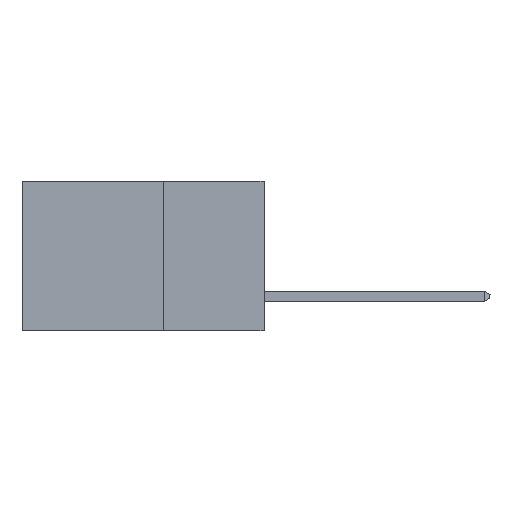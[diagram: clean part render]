
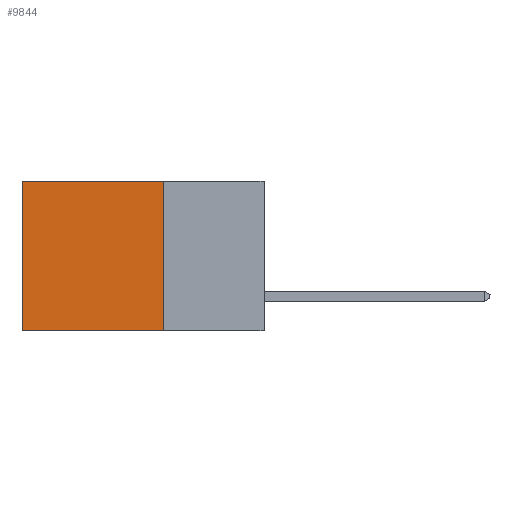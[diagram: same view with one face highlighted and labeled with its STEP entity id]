
A CAD part, left-side view. The second image highlights one B-rep face of the part: STEP entity #9844.
In plain terms, the highlighted planar face has unit normal (-1, 0, 0).
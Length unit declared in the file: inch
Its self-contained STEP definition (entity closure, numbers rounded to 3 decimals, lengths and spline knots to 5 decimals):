
#89 = ORIENTED_EDGE ( 'NONE', *, *, #6728, .F. ) ;
#309 = VERTEX_POINT ( 'NONE', #2510 ) ;
#455 = DIRECTION ( 'NONE',  ( 0., 0., -1. ) ) ;
#757 = DIRECTION ( 'NONE',  ( 0., 0., -1. ) ) ;
#859 = ORIENTED_EDGE ( 'NONE', *, *, #11018, .T. ) ;
#1404 = ORIENTED_EDGE ( 'NONE', *, *, #5015, .F. ) ;
#1527 = LINE ( 'NONE', #5231, #3447 ) ;
#2150 = CARTESIAN_POINT ( 'NONE',  ( 0.2615, 0.6, -0.37 ) ) ;
#2510 = CARTESIAN_POINT ( 'NONE',  ( 0.2615, 0.25, 0. ) ) ;
#2653 = DIRECTION ( 'NONE',  ( 0., 0., -1. ) ) ;
#3284 = FACE_OUTER_BOUND ( 'NONE', #9529, .T. ) ;
#3447 = VECTOR ( 'NONE', #9069, 39.37008 ) ;
#4104 = CARTESIAN_POINT ( 'NONE',  ( 0.2615, 0.6, 0. ) ) ;
#4286 = CARTESIAN_POINT ( 'NONE',  ( 0.2615, 0.25, -0.37 ) ) ;
#4543 = AXIS2_PLACEMENT_3D ( 'NONE', #8297, #9303, #757 ) ;
#4588 = PLANE ( 'NONE',  #4543 ) ;
#5015 = EDGE_CURVE ( 'NONE', #11475, #9988, #1527, .T. ) ;
#5231 = CARTESIAN_POINT ( 'NONE',  ( 0.2615, 0.25, -0.37 ) ) ;
#5339 = VECTOR ( 'NONE', #11025, 39.37008 ) ;
#5340 = LINE ( 'NONE', #4286, #7482 ) ;
#5407 = CARTESIAN_POINT ( 'NONE',  ( 0.2615, 0.25, 0. ) ) ;
#6612 = LINE ( 'NONE', #12159, #7314 ) ;
#6635 = CARTESIAN_POINT ( 'NONE',  ( 0.2615, 0.25, -0.37 ) ) ;
#6728 = EDGE_CURVE ( 'NONE', #309, #11475, #5340, .T. ) ;
#7314 = VECTOR ( 'NONE', #2653, 39.37008 ) ;
#7482 = VECTOR ( 'NONE', #455, 39.37008 ) ;
#8270 = EDGE_CURVE ( 'NONE', #9709, #9988, #6612, .T. ) ;
#8297 = CARTESIAN_POINT ( 'NONE',  ( 0.2615, 0.25, -0.37 ) ) ;
#9069 = DIRECTION ( 'NONE',  ( 0., 1., 0. ) ) ;
#9303 = DIRECTION ( 'NONE',  ( 1., 0., 0. ) ) ;
#9529 = EDGE_LOOP ( 'NONE', ( #12020, #1404, #89, #859 ) ) ;
#9709 = VERTEX_POINT ( 'NONE', #4104 ) ;
#9844 = ADVANCED_FACE ( 'NONE', ( #3284 ), #4588, .F. ) ;
#9988 = VERTEX_POINT ( 'NONE', #2150 ) ;
#11018 = EDGE_CURVE ( 'NONE', #309, #9709, #11141, .T. ) ;
#11025 = DIRECTION ( 'NONE',  ( 0., 1., 0. ) ) ;
#11141 = LINE ( 'NONE', #5407, #5339 ) ;
#11475 = VERTEX_POINT ( 'NONE', #6635 ) ;
#12020 = ORIENTED_EDGE ( 'NONE', *, *, #8270, .T. ) ;
#12159 = CARTESIAN_POINT ( 'NONE',  ( 0.2615, 0.6, -0.37 ) ) ;
